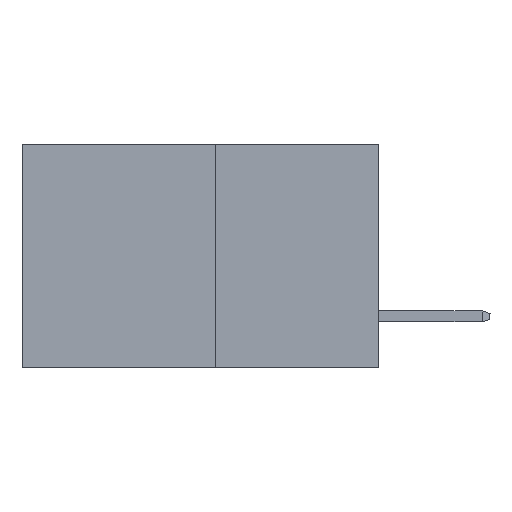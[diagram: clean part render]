
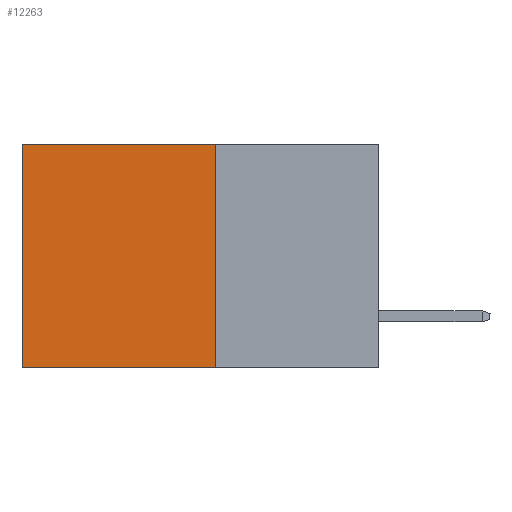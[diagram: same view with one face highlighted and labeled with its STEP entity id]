
A CAD part, left-side view. The second image highlights one B-rep face of the part: STEP entity #12263.
In plain terms, the highlighted planar face has unit normal (-1, 0, 0).
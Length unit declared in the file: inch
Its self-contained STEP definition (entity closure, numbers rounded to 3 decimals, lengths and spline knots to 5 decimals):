
#289 = DIRECTION ( 'NONE',  ( 0., 1., 0. ) ) ;
#333 = EDGE_LOOP ( 'NONE', ( #2576, #2647, #2634, #8797 ) ) ;
#347 = EDGE_CURVE ( 'NONE', #6606, #3797, #9777, .T. ) ;
#411 = EDGE_CURVE ( 'NONE', #6882, #5273, #6653, .T. ) ;
#706 = VECTOR ( 'NONE', #5512, 39.37008 ) ;
#889 = EDGE_CURVE ( 'NONE', #5273, #3797, #11108, .T. ) ;
#1543 = LINE ( 'NONE', #11556, #3423 ) ;
#1844 = CARTESIAN_POINT ( 'NONE',  ( 0.277, 0.59, -0.37 ) ) ;
#2576 = ORIENTED_EDGE ( 'NONE', *, *, #347, .T. ) ;
#2634 = ORIENTED_EDGE ( 'NONE', *, *, #411, .F. ) ;
#2647 = ORIENTED_EDGE ( 'NONE', *, *, #889, .F. ) ;
#2965 = CARTESIAN_POINT ( 'NONE',  ( 0.277, 0.27, -0.37 ) ) ;
#3302 = CARTESIAN_POINT ( 'NONE',  ( 0.277, 0.59, -0.37 ) ) ;
#3423 = VECTOR ( 'NONE', #289, 39.37008 ) ;
#3732 = CARTESIAN_POINT ( 'NONE',  ( 0.277, 0.27, -0.37 ) ) ;
#3797 = VERTEX_POINT ( 'NONE', #3302 ) ;
#3926 = VECTOR ( 'NONE', #7160, 39.37008 ) ;
#4182 = AXIS2_PLACEMENT_3D ( 'NONE', #3732, #10630, #4817 ) ;
#4817 = DIRECTION ( 'NONE',  ( 0., 0., -1. ) ) ;
#5273 = VERTEX_POINT ( 'NONE', #5675 ) ;
#5512 = DIRECTION ( 'NONE',  ( 0., 1., 0. ) ) ;
#5675 = CARTESIAN_POINT ( 'NONE',  ( 0.277, 0.27, -0.37 ) ) ;
#6606 = VERTEX_POINT ( 'NONE', #12507 ) ;
#6653 = LINE ( 'NONE', #2965, #3926 ) ;
#6701 = CARTESIAN_POINT ( 'NONE',  ( 0.277, 0.27, -0.37 ) ) ;
#6882 = VERTEX_POINT ( 'NONE', #11587 ) ;
#7160 = DIRECTION ( 'NONE',  ( 0., 0., -1. ) ) ;
#7252 = EDGE_CURVE ( 'NONE', #6882, #6606, #1543, .T. ) ;
#8797 = ORIENTED_EDGE ( 'NONE', *, *, #7252, .T. ) ;
#9665 = PLANE ( 'NONE',  #4182 ) ;
#9777 = LINE ( 'NONE', #1844, #12029 ) ;
#10150 = FACE_OUTER_BOUND ( 'NONE', #333, .T. ) ;
#10630 = DIRECTION ( 'NONE',  ( 1., 0., 0. ) ) ;
#11108 = LINE ( 'NONE', #6701, #706 ) ;
#11556 = CARTESIAN_POINT ( 'NONE',  ( 0.277, 0.27, 0. ) ) ;
#11587 = CARTESIAN_POINT ( 'NONE',  ( 0.277, 0.27, 0. ) ) ;
#11866 = DIRECTION ( 'NONE',  ( 0., 0., -1. ) ) ;
#12029 = VECTOR ( 'NONE', #11866, 39.37008 ) ;
#12263 = ADVANCED_FACE ( 'NONE', ( #10150 ), #9665, .F. ) ;
#12507 = CARTESIAN_POINT ( 'NONE',  ( 0.277, 0.59, 0. ) ) ;
